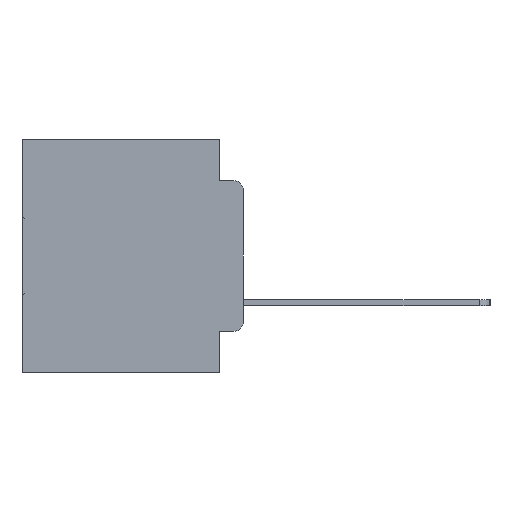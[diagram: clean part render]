
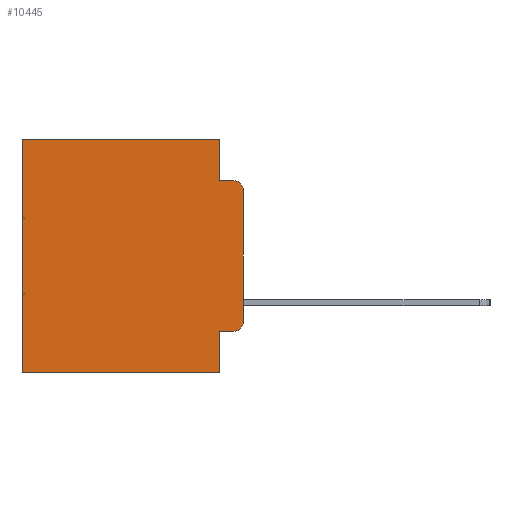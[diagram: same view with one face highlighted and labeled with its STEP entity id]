
A CAD part, left-side view. The second image highlights one B-rep face of the part: STEP entity #10445.
In plain terms, the highlighted planar face has unit normal (-1, 0, 0).
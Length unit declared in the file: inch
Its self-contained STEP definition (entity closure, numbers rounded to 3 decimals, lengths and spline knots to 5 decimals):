
#474 = CARTESIAN_POINT ( 'NONE',  ( 0.298, 0.051, -0.5 ) ) ;
#1036 = ORIENTED_EDGE ( 'NONE', *, *, #24347, .T. ) ;
#1079 = CARTESIAN_POINT ( 'NONE',  ( 0.298, 0., -0.5 ) ) ;
#1201 = CIRCLE ( 'NONE', #30621, 0.02 ) ;
#1365 = CARTESIAN_POINT ( 'NONE',  ( 0.298, 0.051, -0.0885 ) ) ;
#1384 = DIRECTION ( 'NONE',  ( 0., 0., -1. ) ) ;
#1563 = EDGE_CURVE ( 'NONE', #22353, #18510, #4278, .T. ) ;
#1689 = CARTESIAN_POINT ( 'NONE',  ( 0.298, 0., -0.3915 ) ) ;
#1831 = CARTESIAN_POINT ( 'NONE',  ( 0.298, 0.473, 0. ) ) ;
#2132 = VERTEX_POINT ( 'NONE', #24947 ) ;
#2652 = VERTEX_POINT ( 'NONE', #1689 ) ;
#3179 = LINE ( 'NONE', #21372, #28501 ) ;
#3300 = EDGE_CURVE ( 'NONE', #23221, #22158, #32449, .T. ) ;
#3604 = DIRECTION ( 'NONE',  ( 0., 0., -1. ) ) ;
#4278 = LINE ( 'NONE', #20255, #30285 ) ;
#5002 = DIRECTION ( 'NONE',  ( 0., 0., -1. ) ) ;
#5691 = VERTEX_POINT ( 'NONE', #23565 ) ;
#6726 = DIRECTION ( 'NONE',  ( 0., 1., 0. ) ) ;
#7917 = ORIENTED_EDGE ( 'NONE', *, *, #12467, .F. ) ;
#8694 = ORIENTED_EDGE ( 'NONE', *, *, #28378, .T. ) ;
#8750 = VERTEX_POINT ( 'NONE', #14065 ) ;
#9229 = LINE ( 'NONE', #1079, #16741 ) ;
#9304 = CARTESIAN_POINT ( 'NONE',  ( 0.298, 0.02, -0.0885 ) ) ;
#10317 = EDGE_CURVE ( 'NONE', #2132, #11868, #12649, .T. ) ;
#10445 = ADVANCED_FACE ( 'NONE', ( #21173 ), #23258, .F. ) ;
#10922 = CIRCLE ( 'NONE', #20649, 0.02 ) ;
#11105 = EDGE_LOOP ( 'NONE', ( #29044, #15078, #20898, #24843, #8694, #11988, #7917, #25694, #31782, #1036 ) ) ;
#11868 = VERTEX_POINT ( 'NONE', #1365 ) ;
#11988 = ORIENTED_EDGE ( 'NONE', *, *, #3300, .T. ) ;
#12171 = DIRECTION ( 'NONE',  ( 0., 0., -1. ) ) ;
#12467 = EDGE_CURVE ( 'NONE', #18510, #22158, #9229, .T. ) ;
#12649 = LINE ( 'NONE', #30183, #18474 ) ;
#13358 = DIRECTION ( 'NONE',  ( 1., 0., 0. ) ) ;
#13610 = CARTESIAN_POINT ( 'NONE',  ( 0.298, 0.473, -0.5 ) ) ;
#13986 = DIRECTION ( 'NONE',  ( 0., 1., 0. ) ) ;
#14065 = CARTESIAN_POINT ( 'NONE',  ( 0.298, 0.02, -0.4115 ) ) ;
#14489 = CARTESIAN_POINT ( 'NONE',  ( 0.298, 0.051, -0.4115 ) ) ;
#14568 = VECTOR ( 'NONE', #6726, 39.37008 ) ;
#14734 = DIRECTION ( 'NONE',  ( -1., 0., 0. ) ) ;
#15078 = ORIENTED_EDGE ( 'NONE', *, *, #17040, .T. ) ;
#15320 = DIRECTION ( 'NONE',  ( 0., -1., 0. ) ) ;
#15383 = CARTESIAN_POINT ( 'NONE',  ( 0.298, 0.051, -0.0885 ) ) ;
#15385 = LINE ( 'NONE', #15383, #21166 ) ;
#15400 = EDGE_CURVE ( 'NONE', #11868, #32518, #15385, .T. ) ;
#16741 = VECTOR ( 'NONE', #13986, 39.37008 ) ;
#16770 = DIRECTION ( 'NONE',  ( -1., 0., 0. ) ) ;
#16898 = AXIS2_PLACEMENT_3D ( 'NONE', #30619, #13358, #30722 ) ;
#17040 = EDGE_CURVE ( 'NONE', #5691, #32518, #10922, .T. ) ;
#18474 = VECTOR ( 'NONE', #5002, 39.37008 ) ;
#18510 = VERTEX_POINT ( 'NONE', #474 ) ;
#19274 = VECTOR ( 'NONE', #12171, 39.37008 ) ;
#20255 = CARTESIAN_POINT ( 'NONE',  ( 0.298, 0.051, 0. ) ) ;
#20649 = AXIS2_PLACEMENT_3D ( 'NONE', #29599, #14734, #32027 ) ;
#20898 = ORIENTED_EDGE ( 'NONE', *, *, #15400, .F. ) ;
#21132 = LINE ( 'NONE', #21863, #14568 ) ;
#21166 = VECTOR ( 'NONE', #30341, 39.37008 ) ;
#21173 = FACE_OUTER_BOUND ( 'NONE', #11105, .T. ) ;
#21372 = CARTESIAN_POINT ( 'NONE',  ( 0.298, 0., 0. ) ) ;
#21863 = CARTESIAN_POINT ( 'NONE',  ( 0.298, 0., 0. ) ) ;
#22158 = VERTEX_POINT ( 'NONE', #13610 ) ;
#22353 = VERTEX_POINT ( 'NONE', #14489 ) ;
#22708 = CARTESIAN_POINT ( 'NONE',  ( 0.298, 0.051, -0.4115 ) ) ;
#23019 = CARTESIAN_POINT ( 'NONE',  ( 0.298, 0.473, 0. ) ) ;
#23221 = VERTEX_POINT ( 'NONE', #23019 ) ;
#23258 = PLANE ( 'NONE',  #16898 ) ;
#23565 = CARTESIAN_POINT ( 'NONE',  ( 0.298, 0., -0.1085 ) ) ;
#24347 = EDGE_CURVE ( 'NONE', #8750, #2652, #1201, .T. ) ;
#24621 = VECTOR ( 'NONE', #15320, 39.37008 ) ;
#24843 = ORIENTED_EDGE ( 'NONE', *, *, #10317, .F. ) ;
#24947 = CARTESIAN_POINT ( 'NONE',  ( 0.298, 0.051, 0. ) ) ;
#25406 = EDGE_CURVE ( 'NONE', #5691, #2652, #3179, .T. ) ;
#25694 = ORIENTED_EDGE ( 'NONE', *, *, #1563, .F. ) ;
#28378 = EDGE_CURVE ( 'NONE', #2132, #23221, #21132, .T. ) ;
#28501 = VECTOR ( 'NONE', #3604, 39.37008 ) ;
#29044 = ORIENTED_EDGE ( 'NONE', *, *, #25406, .F. ) ;
#29321 = EDGE_CURVE ( 'NONE', #22353, #8750, #31919, .T. ) ;
#29599 = CARTESIAN_POINT ( 'NONE',  ( 0.298, 0.02, -0.1085 ) ) ;
#30137 = DIRECTION ( 'NONE',  ( 0., 0., -1. ) ) ;
#30183 = CARTESIAN_POINT ( 'NONE',  ( 0.298, 0.051, 0. ) ) ;
#30285 = VECTOR ( 'NONE', #30137, 39.37008 ) ;
#30341 = DIRECTION ( 'NONE',  ( 0., -1., 0. ) ) ;
#30619 = CARTESIAN_POINT ( 'NONE',  ( 0.298, 0., 0. ) ) ;
#30621 = AXIS2_PLACEMENT_3D ( 'NONE', #31608, #16770, #1384 ) ;
#30722 = DIRECTION ( 'NONE',  ( 0., 0., -1. ) ) ;
#31608 = CARTESIAN_POINT ( 'NONE',  ( 0.298, 0.02, -0.3915 ) ) ;
#31782 = ORIENTED_EDGE ( 'NONE', *, *, #29321, .T. ) ;
#31919 = LINE ( 'NONE', #22708, #24621 ) ;
#32027 = DIRECTION ( 'NONE',  ( 0., 0., -1. ) ) ;
#32449 = LINE ( 'NONE', #1831, #19274 ) ;
#32518 = VERTEX_POINT ( 'NONE', #9304 ) ;
